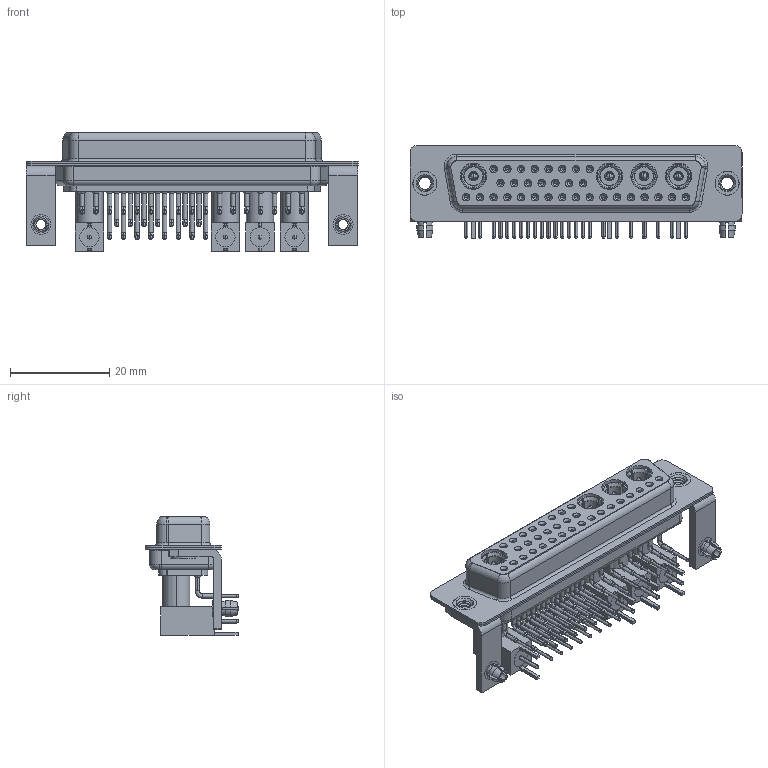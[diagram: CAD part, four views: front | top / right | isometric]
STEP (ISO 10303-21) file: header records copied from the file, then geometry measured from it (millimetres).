
FILE_DESCRIPTION (( 'STEP AP203' ), '1' );
FILE_NAME ('630-36W4240-7NB.STEP', '2022-06-09T08:28:51', ( '' ), ( '' ), 'SwSTEP 2.0', 'SolidWorks 2020', '' );
FILE_SCHEMA (( 'CONFIG_CONTROL_DESIGN' ));
Length unit declared in the file: millimetre
Products named in the file (20): RA Back Shell_50; Locking Collar; Co-Ax Plug Assy_RA 50; Insulator Pin_Straight PC Tail; 630Combo Shell Front_50 Contacts; Co-Ax Plug_RA 50; 630Combo Contact Row 1_50 Contacts; 630Combo Contact Row 2_50 Contacts; 630Combo Threaded Rivet_B; 630-36W4240-7NB; 630Combo Housing_36W4; Insulator RA Pin; 630Combo Contact Row 3; 630Combo Board Lock_50 Contacts; 630Combo Shell Rear_50 Contacts; Pin_RA 50; 630Combo Stabilizer Bracket_50 Contacts
Assembly tree (69 placements, depth 3):
  630-36W4240-7NB
    630Combo Housing_36W4
    630Combo Shell Front_50 Contacts
    630Combo Shell Rear_50 Contacts
    630Combo Threaded Rivet_B  x2
    630Combo Stabilizer Bracket_50 Contacts  x2
    630Combo Board Lock_50 Contacts  x2
    Co-Ax Plug Assy_RA 50
      Co-Ax Plug_RA 50
      Insulator Pin_Straight PC Tail
      Pin_RA 50
      Locking Collar
      RA Back Shell_50
      Insulator RA Pin
    Co-Ax Plug Assy_RA 50
      Co-Ax Plug_RA 50
      Insulator Pin_Straight PC Tail
      Pin_RA 50
      Locking Collar
      RA Back Shell_50
      Insulator RA Pin
    Co-Ax Plug Assy_RA 50
      Co-Ax Plug_RA 50
      Insulator Pin_Straight PC Tail
      Pin_RA 50
      Locking Collar
      RA Back Shell_50
      Insulator RA Pin
    Co-Ax Plug Assy_RA 50
      Co-Ax Plug_RA 50
      Insulator Pin_Straight PC Tail
      Pin_RA 50
      Locking Collar
      RA Back Shell_50
      Insulator RA Pin
    630Combo Contact Row 1_50 Contacts  x8
    630Combo Contact Row 2_50 Contacts  x7
    630Combo Contact Row 3  x17
Bounding box: 67 x 18.8 x 23.95 mm (x, y, z)
Volume: 8673.2 mm3; surface area: 19610.8 mm2
Topology: 65 solids, 65 shells, 2777 faces, 6953 edges, 4377 vertices
Faces by surface type: cylinder 1183, plane 883, cone 476, bspline 138, torus 81, sphere 16
Entity records: 35566 total; most frequent: CARTESIAN_POINT 7197, DIRECTION 5751, ORIENTED_EDGE 4812, EDGE_CURVE 2406, AXIS2_PLACEMENT_3D 2382, VERTEX_POINT 1538, CIRCLE 1292, EDGE_LOOP 1262
